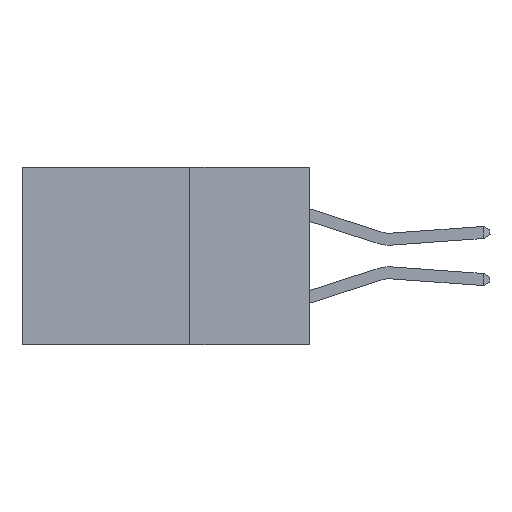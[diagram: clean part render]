
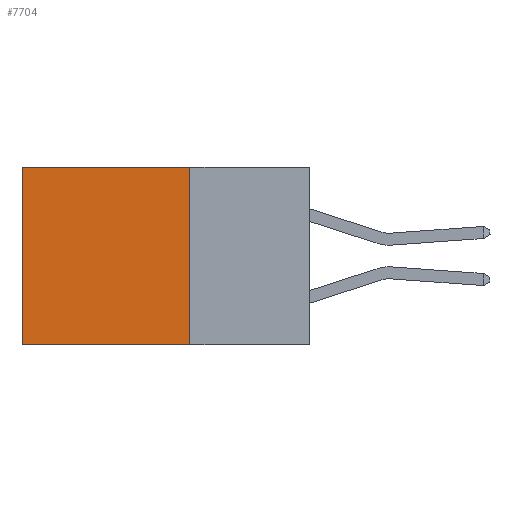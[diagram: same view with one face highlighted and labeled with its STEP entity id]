
A CAD part, left-side view. The second image highlights one B-rep face of the part: STEP entity #7704.
In plain terms, the highlighted planar face has unit normal (-1, 0, 0).
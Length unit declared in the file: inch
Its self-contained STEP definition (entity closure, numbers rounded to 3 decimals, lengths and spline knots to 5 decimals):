
#261 = VERTEX_POINT ( 'NONE', #4994 ) ;
#419 = VECTOR ( 'NONE', #14293, 39.37008 ) ;
#475 = LINE ( 'NONE', #7979, #419 ) ;
#500 = ORIENTED_EDGE ( 'NONE', *, *, #7866, .T. ) ;
#2301 = VERTEX_POINT ( 'NONE', #2385 ) ;
#2385 = CARTESIAN_POINT ( 'NONE',  ( 0.2615, 0.6, 0. ) ) ;
#2561 = DIRECTION ( 'NONE',  ( 0., 1., 0. ) ) ;
#3821 = LINE ( 'NONE', #8862, #7534 ) ;
#3964 = VECTOR ( 'NONE', #7679, 39.37008 ) ;
#4389 = FACE_OUTER_BOUND ( 'NONE', #5374, .T. ) ;
#4994 = CARTESIAN_POINT ( 'NONE',  ( 0.2615, 0.25, 0. ) ) ;
#5268 = PLANE ( 'NONE',  #13183 ) ;
#5374 = EDGE_LOOP ( 'NONE', ( #6399, #13690, #7620, #500 ) ) ;
#5401 = CARTESIAN_POINT ( 'NONE',  ( 0.2615, 0.25, -0.37 ) ) ;
#6338 = VERTEX_POINT ( 'NONE', #6693 ) ;
#6369 = CARTESIAN_POINT ( 'NONE',  ( 0.2615, 0.25, 0. ) ) ;
#6399 = ORIENTED_EDGE ( 'NONE', *, *, #14208, .T. ) ;
#6693 = CARTESIAN_POINT ( 'NONE',  ( 0.2615, 0.6, -0.37 ) ) ;
#7050 = VECTOR ( 'NONE', #11550, 39.37008 ) ;
#7534 = VECTOR ( 'NONE', #2561, 39.37008 ) ;
#7620 = ORIENTED_EDGE ( 'NONE', *, *, #13409, .F. ) ;
#7679 = DIRECTION ( 'NONE',  ( 0., 1., 0. ) ) ;
#7704 = ADVANCED_FACE ( 'NONE', ( #4389 ), #5268, .F. ) ;
#7866 = EDGE_CURVE ( 'NONE', #261, #2301, #12591, .T. ) ;
#7979 = CARTESIAN_POINT ( 'NONE',  ( 0.2615, 0.25, -0.37 ) ) ;
#8086 = DIRECTION ( 'NONE',  ( 1., 0., 0. ) ) ;
#8862 = CARTESIAN_POINT ( 'NONE',  ( 0.2615, 0.25, -0.37 ) ) ;
#9032 = VERTEX_POINT ( 'NONE', #5401 ) ;
#10263 = LINE ( 'NONE', #13750, #7050 ) ;
#10324 = DIRECTION ( 'NONE',  ( 0., 0., -1. ) ) ;
#11550 = DIRECTION ( 'NONE',  ( 0., 0., -1. ) ) ;
#12591 = LINE ( 'NONE', #6369, #3964 ) ;
#12889 = EDGE_CURVE ( 'NONE', #9032, #6338, #3821, .T. ) ;
#13183 = AXIS2_PLACEMENT_3D ( 'NONE', #15376, #8086, #10324 ) ;
#13409 = EDGE_CURVE ( 'NONE', #261, #9032, #475, .T. ) ;
#13690 = ORIENTED_EDGE ( 'NONE', *, *, #12889, .F. ) ;
#13750 = CARTESIAN_POINT ( 'NONE',  ( 0.2615, 0.6, -0.37 ) ) ;
#14208 = EDGE_CURVE ( 'NONE', #2301, #6338, #10263, .T. ) ;
#14293 = DIRECTION ( 'NONE',  ( 0., 0., -1. ) ) ;
#15376 = CARTESIAN_POINT ( 'NONE',  ( 0.2615, 0.25, -0.37 ) ) ;
